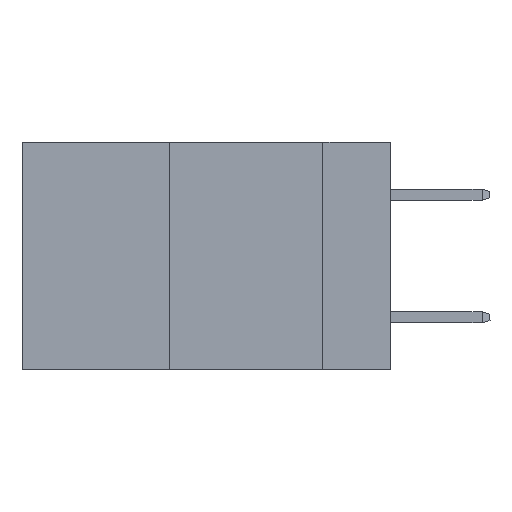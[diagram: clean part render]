
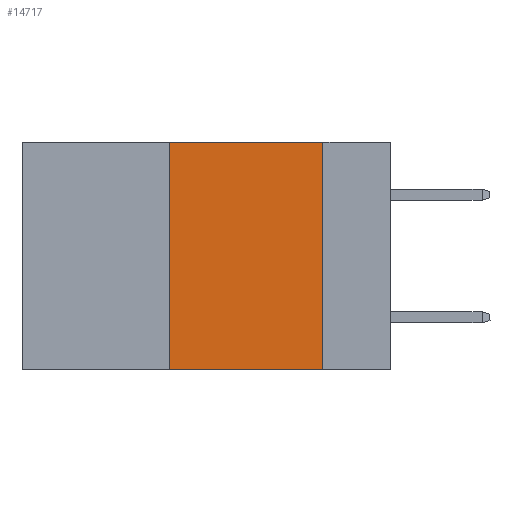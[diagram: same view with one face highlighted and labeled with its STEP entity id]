
A CAD part, left-side view. The second image highlights one B-rep face of the part: STEP entity #14717.
In plain terms, the highlighted planar face has unit normal (-1, 0, 0).
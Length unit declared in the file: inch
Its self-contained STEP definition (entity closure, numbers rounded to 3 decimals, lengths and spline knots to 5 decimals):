
#131 = DIRECTION ( 'NONE',  ( 0., 0., 1. ) ) ;
#655 = CARTESIAN_POINT ( 'NONE',  ( 0., 0.11, -0.37 ) ) ;
#805 = ORIENTED_EDGE ( 'NONE', *, *, #9817, .T. ) ;
#972 = EDGE_LOOP ( 'NONE', ( #7541, #14598, #5729, #805 ) ) ;
#1046 = VERTEX_POINT ( 'NONE', #655 ) ;
#1225 = DIRECTION ( 'NONE',  ( 1., 0., 0. ) ) ;
#1652 = VECTOR ( 'NONE', #15388, 39.37008 ) ;
#1832 = CARTESIAN_POINT ( 'NONE',  ( 0., 0.6, -0.37 ) ) ;
#3809 = CARTESIAN_POINT ( 'NONE',  ( 0., 0.36, 0. ) ) ;
#4575 = EDGE_CURVE ( 'NONE', #13538, #15423, #13425, .T. ) ;
#5729 = ORIENTED_EDGE ( 'NONE', *, *, #13550, .F. ) ;
#5894 = DIRECTION ( 'NONE',  ( 0., -1., 0. ) ) ;
#6161 = AXIS2_PLACEMENT_3D ( 'NONE', #8682, #1225, #7373 ) ;
#6211 = VECTOR ( 'NONE', #5894, 39.37008 ) ;
#6307 = LINE ( 'NONE', #8748, #8071 ) ;
#7105 = CARTESIAN_POINT ( 'NONE',  ( 0., 0.6, 0. ) ) ;
#7146 = PLANE ( 'NONE',  #6161 ) ;
#7373 = DIRECTION ( 'NONE',  ( 0., 0., -1. ) ) ;
#7541 = ORIENTED_EDGE ( 'NONE', *, *, #7960, .F. ) ;
#7960 = EDGE_CURVE ( 'NONE', #15423, #1046, #11763, .T. ) ;
#8071 = VECTOR ( 'NONE', #131, 39.37008 ) ;
#8305 = CARTESIAN_POINT ( 'NONE',  ( 0., 0.11, 0. ) ) ;
#8682 = CARTESIAN_POINT ( 'NONE',  ( 0., 0.6, 0. ) ) ;
#8748 = CARTESIAN_POINT ( 'NONE',  ( 0., 0.36, 0. ) ) ;
#9197 = VECTOR ( 'NONE', #15671, 39.37008 ) ;
#9817 = EDGE_CURVE ( 'NONE', #15454, #1046, #15313, .T. ) ;
#9918 = FACE_OUTER_BOUND ( 'NONE', #972, .T. ) ;
#11763 = LINE ( 'NONE', #13060, #9197 ) ;
#13060 = CARTESIAN_POINT ( 'NONE',  ( 0., 0.11, 0. ) ) ;
#13425 = LINE ( 'NONE', #7105, #6211 ) ;
#13538 = VERTEX_POINT ( 'NONE', #3809 ) ;
#13550 = EDGE_CURVE ( 'NONE', #15454, #13538, #6307, .T. ) ;
#14387 = CARTESIAN_POINT ( 'NONE',  ( 0., 0.36, -0.37 ) ) ;
#14598 = ORIENTED_EDGE ( 'NONE', *, *, #4575, .F. ) ;
#14717 = ADVANCED_FACE ( 'NONE', ( #9918 ), #7146, .F. ) ;
#15313 = LINE ( 'NONE', #1832, #1652 ) ;
#15388 = DIRECTION ( 'NONE',  ( 0., -1., 0. ) ) ;
#15423 = VERTEX_POINT ( 'NONE', #8305 ) ;
#15454 = VERTEX_POINT ( 'NONE', #14387 ) ;
#15671 = DIRECTION ( 'NONE',  ( 0., 0., -1. ) ) ;
